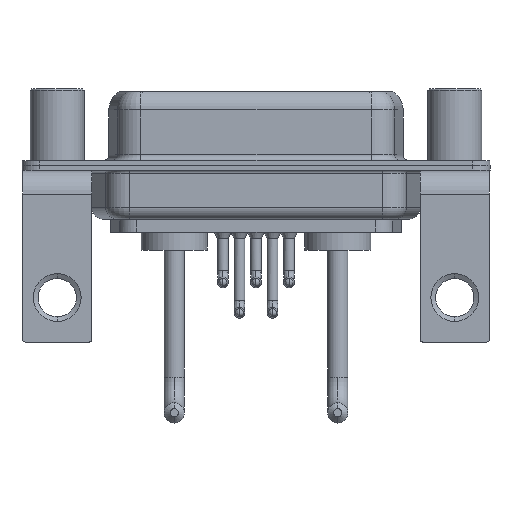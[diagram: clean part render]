
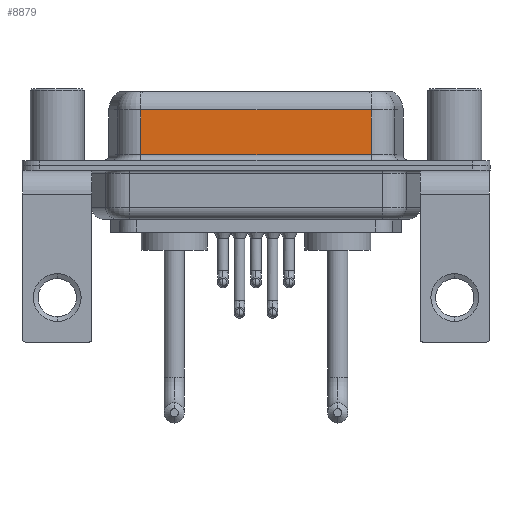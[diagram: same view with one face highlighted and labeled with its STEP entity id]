
A CAD part, front view. The second image highlights one B-rep face of the part: STEP entity #8879.
In plain terms, the highlighted planar face has unit normal (0, -1, 0).
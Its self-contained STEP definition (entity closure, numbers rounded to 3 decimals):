
#40 = DIRECTION ( 'NONE',  ( 0., 1., 0. ) ) ;
#118 = VECTOR ( 'NONE', #9213, 1000. ) ;
#636 = ORIENTED_EDGE ( 'NONE', *, *, #13569, .F. ) ;
#703 = LINE ( 'NONE', #5123, #5899 ) ;
#1005 = CARTESIAN_POINT ( 'NONE',  ( 26.287, -3.95, 0.9 ) ) ;
#2606 = EDGE_CURVE ( 'NONE', #4538, #18558, #11498, .T. ) ;
#3101 = FACE_OUTER_BOUND ( 'NONE', #14642, .T. ) ;
#3200 = CARTESIAN_POINT ( 'NONE',  ( 26.287, -3.95, 6.4 ) ) ;
#3315 = ORIENTED_EDGE ( 'NONE', *, *, #2606, .T. ) ;
#3707 = CARTESIAN_POINT ( 'NONE',  ( 7.013, -3.95, 0.9 ) ) ;
#4538 = VERTEX_POINT ( 'NONE', #13497 ) ;
#4770 = PLANE ( 'NONE',  #12916 ) ;
#5123 = CARTESIAN_POINT ( 'NONE',  ( 26.287, -3.95, 4.65 ) ) ;
#5808 = VECTOR ( 'NONE', #17746, 1000. ) ;
#5899 = VECTOR ( 'NONE', #17189, 1000. ) ;
#6058 = DIRECTION ( 'NONE',  ( 0., 0., 1. ) ) ;
#6383 = CARTESIAN_POINT ( 'NONE',  ( 26.287, -3.95, 4.65 ) ) ;
#6412 = ORIENTED_EDGE ( 'NONE', *, *, #16726, .T. ) ;
#8879 = ADVANCED_FACE ( 'NONE', ( #3101 ), #4770, .F. ) ;
#9213 = DIRECTION ( 'NONE',  ( 0., 0., -1. ) ) ;
#11151 = CARTESIAN_POINT ( 'NONE',  ( 26.287, -3.95, 0.9 ) ) ;
#11498 = LINE ( 'NONE', #13236, #5808 ) ;
#12016 = VERTEX_POINT ( 'NONE', #11151 ) ;
#12916 = AXIS2_PLACEMENT_3D ( 'NONE', #19381, #40, #6058 ) ;
#13135 = VERTEX_POINT ( 'NONE', #6383 ) ;
#13236 = CARTESIAN_POINT ( 'NONE',  ( 7.013, -3.95, 6.4 ) ) ;
#13497 = CARTESIAN_POINT ( 'NONE',  ( 7.013, -3.95, 4.65 ) ) ;
#13569 = EDGE_CURVE ( 'NONE', #13135, #12016, #14003, .T. ) ;
#14003 = LINE ( 'NONE', #3200, #118 ) ;
#14253 = DIRECTION ( 'NONE',  ( 1., 0., 0. ) ) ;
#14642 = EDGE_LOOP ( 'NONE', ( #636, #6412, #3315, #19231 ) ) ;
#15576 = VECTOR ( 'NONE', #14253, 1000. ) ;
#16726 = EDGE_CURVE ( 'NONE', #13135, #4538, #703, .T. ) ;
#17189 = DIRECTION ( 'NONE',  ( -1., 0., 0. ) ) ;
#17599 = EDGE_CURVE ( 'NONE', #18558, #12016, #18668, .T. ) ;
#17746 = DIRECTION ( 'NONE',  ( 0., 0., -1. ) ) ;
#18558 = VERTEX_POINT ( 'NONE', #3707 ) ;
#18668 = LINE ( 'NONE', #1005, #15576 ) ;
#19231 = ORIENTED_EDGE ( 'NONE', *, *, #17599, .T. ) ;
#19381 = CARTESIAN_POINT ( 'NONE',  ( 26.287, -3.95, 6.4 ) ) ;
